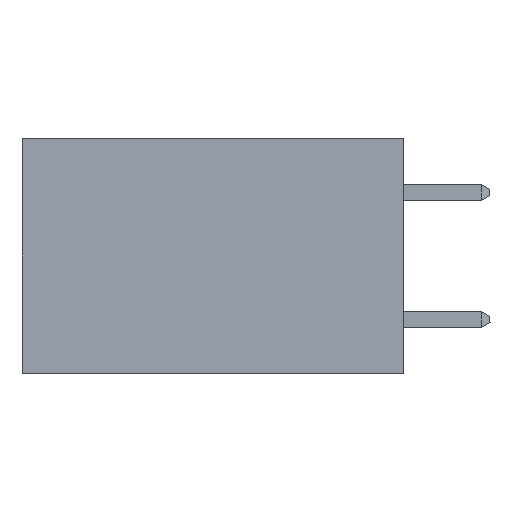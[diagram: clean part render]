
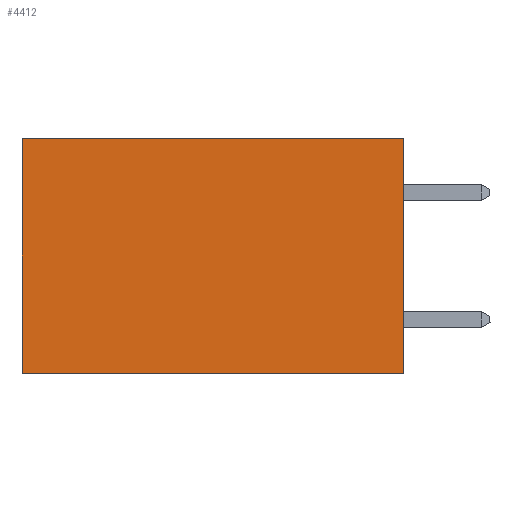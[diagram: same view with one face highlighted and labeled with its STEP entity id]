
A CAD part, left-side view. The second image highlights one B-rep face of the part: STEP entity #4412.
In plain terms, the highlighted planar face has unit normal (-1, 0, 0).
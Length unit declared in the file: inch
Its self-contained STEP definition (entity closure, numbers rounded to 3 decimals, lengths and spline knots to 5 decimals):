
#433 = CARTESIAN_POINT ( 'NONE',  ( 0.2875, 0.6, -0.37 ) ) ;
#489 = VERTEX_POINT ( 'NONE', #19349 ) ;
#1150 = VECTOR ( 'NONE', #12000, 39.37008 ) ;
#2789 = ORIENTED_EDGE ( 'NONE', *, *, #32043, .F. ) ;
#3076 = PLANE ( 'NONE',  #26375 ) ;
#3962 = EDGE_LOOP ( 'NONE', ( #41105, #2789, #29101, #39504 ) ) ;
#4412 = ADVANCED_FACE ( 'NONE', ( #24801 ), #3076, .F. ) ;
#9310 = CARTESIAN_POINT ( 'NONE',  ( 0.2875, 0., -0.37 ) ) ;
#9331 = VERTEX_POINT ( 'NONE', #10337 ) ;
#10129 = EDGE_CURVE ( 'NONE', #9331, #41786, #31765, .T. ) ;
#10337 = CARTESIAN_POINT ( 'NONE',  ( 0.2875, 0.6, 0. ) ) ;
#10829 = CARTESIAN_POINT ( 'NONE',  ( 0.2875, 0., 0. ) ) ;
#12000 = DIRECTION ( 'NONE',  ( 0., 0., -1. ) ) ;
#12553 = LINE ( 'NONE', #16681, #36172 ) ;
#13399 = DIRECTION ( 'NONE',  ( 1., 0., 0. ) ) ;
#14565 = LINE ( 'NONE', #10829, #32825 ) ;
#15937 = DIRECTION ( 'NONE',  ( 0., 1., 0. ) ) ;
#16681 = CARTESIAN_POINT ( 'NONE',  ( 0.2875, 0., 0. ) ) ;
#19349 = CARTESIAN_POINT ( 'NONE',  ( 0.2875, 0., -0.37 ) ) ;
#20321 = DIRECTION ( 'NONE',  ( 0., 0., -1. ) ) ;
#24109 = VERTEX_POINT ( 'NONE', #36138 ) ;
#24801 = FACE_OUTER_BOUND ( 'NONE', #3962, .T. ) ;
#25021 = EDGE_CURVE ( 'NONE', #24109, #9331, #12553, .T. ) ;
#25261 = LINE ( 'NONE', #9310, #37559 ) ;
#26375 = AXIS2_PLACEMENT_3D ( 'NONE', #37504, #13399, #20321 ) ;
#29101 = ORIENTED_EDGE ( 'NONE', *, *, #39054, .F. ) ;
#31765 = LINE ( 'NONE', #42449, #1150 ) ;
#32043 = EDGE_CURVE ( 'NONE', #489, #41786, #25261, .T. ) ;
#32825 = VECTOR ( 'NONE', #34839, 39.37008 ) ;
#34839 = DIRECTION ( 'NONE',  ( 0., 0., -1. ) ) ;
#36138 = CARTESIAN_POINT ( 'NONE',  ( 0.2875, 0., 0. ) ) ;
#36172 = VECTOR ( 'NONE', #37631, 39.37008 ) ;
#37504 = CARTESIAN_POINT ( 'NONE',  ( 0.2875, 0., 0. ) ) ;
#37559 = VECTOR ( 'NONE', #15937, 39.37008 ) ;
#37631 = DIRECTION ( 'NONE',  ( 0., 1., 0. ) ) ;
#39054 = EDGE_CURVE ( 'NONE', #24109, #489, #14565, .T. ) ;
#39504 = ORIENTED_EDGE ( 'NONE', *, *, #25021, .T. ) ;
#41105 = ORIENTED_EDGE ( 'NONE', *, *, #10129, .T. ) ;
#41786 = VERTEX_POINT ( 'NONE', #433 ) ;
#42449 = CARTESIAN_POINT ( 'NONE',  ( 0.2875, 0.6, 0. ) ) ;
